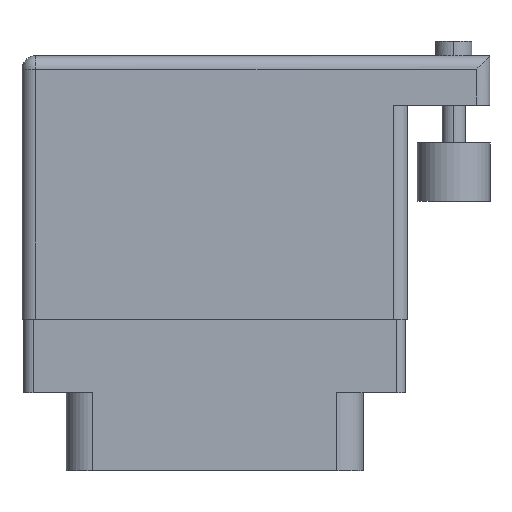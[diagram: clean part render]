
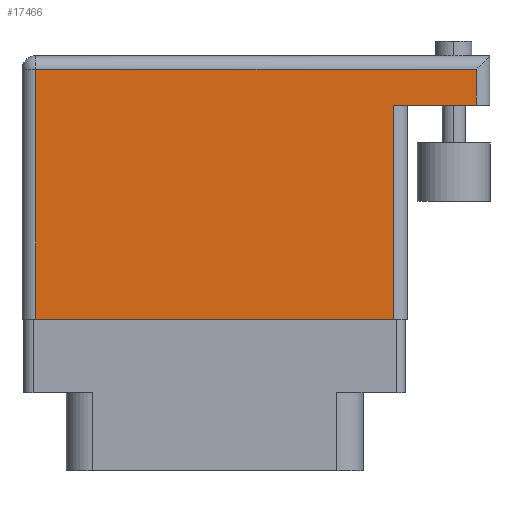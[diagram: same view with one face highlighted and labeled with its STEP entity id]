
A CAD part, front view. The second image highlights one B-rep face of the part: STEP entity #17466.
In plain terms, the highlighted face is planar.
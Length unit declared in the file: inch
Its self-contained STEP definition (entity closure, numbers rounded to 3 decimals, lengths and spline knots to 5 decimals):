
#4 = ORIENTED_EDGE ( 'NONE', *, *, #3222, .T. ) ;
#119 = DIRECTION ( 'NONE',  ( -1., 0., 0. ) ) ;
#309 = LINE ( 'NONE', #24208, #13355 ) ;
#433 = LINE ( 'NONE', #7741, #1077 ) ;
#990 = CARTESIAN_POINT ( 'NONE',  ( 1.562, 0.859, 0. ) ) ;
#1077 = VECTOR ( 'NONE', #3907, 39.37008 ) ;
#1354 = CARTESIAN_POINT ( 'NONE',  ( 1.609, 0.736, 0. ) ) ;
#1380 = CARTESIAN_POINT ( 'NONE',  ( 0., 0., 0. ) ) ;
#1875 = VECTOR ( 'NONE', #16314, 39.37008 ) ;
#2774 = DIRECTION ( 'NONE',  ( 0., 0., -1. ) ) ;
#3222 = EDGE_CURVE ( 'NONE', #6433, #5989, #10558, .T. ) ;
#3278 = ORIENTED_EDGE ( 'NONE', *, *, #6228, .T. ) ;
#3907 = DIRECTION ( 'NONE',  ( 0., -1., 0. ) ) ;
#4564 = PLANE ( 'NONE',  #9302 ) ;
#5813 = VECTOR ( 'NONE', #10812, 39.37008 ) ;
#5989 = VERTEX_POINT ( 'NONE', #990 ) ;
#6154 = EDGE_CURVE ( 'NONE', #6433, #10417, #8744, .T. ) ;
#6228 = EDGE_CURVE ( 'NONE', #17178, #23365, #433, .T. ) ;
#6433 = VERTEX_POINT ( 'NONE', #22819 ) ;
#7741 = CARTESIAN_POINT ( 'NONE',  ( 0.047, 0., 0. ) ) ;
#8744 = LINE ( 'NONE', #1354, #16030 ) ;
#8870 = ORIENTED_EDGE ( 'NONE', *, *, #23609, .T. ) ;
#9105 = EDGE_CURVE ( 'NONE', #5989, #17178, #309, .T. ) ;
#9302 = AXIS2_PLACEMENT_3D ( 'NONE', #12828, #2774, #24795 ) ;
#9848 = CARTESIAN_POINT ( 'NONE',  ( 1.278, 0., 0. ) ) ;
#10344 = CARTESIAN_POINT ( 'NONE',  ( 1.278, 0.736, 0. ) ) ;
#10417 = VERTEX_POINT ( 'NONE', #17077 ) ;
#10509 = ORIENTED_EDGE ( 'NONE', *, *, #9105, .T. ) ;
#10558 = LINE ( 'NONE', #16950, #5813 ) ;
#10812 = DIRECTION ( 'NONE',  ( 0., 1., 0. ) ) ;
#11589 = EDGE_LOOP ( 'NONE', ( #18604, #8870, #24326, #4, #10509, #3278 ) ) ;
#12704 = LINE ( 'NONE', #10344, #1875 ) ;
#12828 = CARTESIAN_POINT ( 'NONE',  ( 0., 0.906, 0. ) ) ;
#13355 = VECTOR ( 'NONE', #119, 39.37008 ) ;
#13416 = CARTESIAN_POINT ( 'NONE',  ( 0.047, 0., 0. ) ) ;
#15413 = DIRECTION ( 'NONE',  ( 1., 0., 0. ) ) ;
#16030 = VECTOR ( 'NONE', #19733, 39.37008 ) ;
#16314 = DIRECTION ( 'NONE',  ( 0., 1., 0. ) ) ;
#16950 = CARTESIAN_POINT ( 'NONE',  ( 1.562, 0.906, 0. ) ) ;
#17077 = CARTESIAN_POINT ( 'NONE',  ( 1.278, 0.736, 0. ) ) ;
#17178 = VERTEX_POINT ( 'NONE', #19935 ) ;
#17466 = ADVANCED_FACE ( 'NONE', ( #19651 ), #4564, .F. ) ;
#18604 = ORIENTED_EDGE ( 'NONE', *, *, #18943, .T. ) ;
#18943 = EDGE_CURVE ( 'NONE', #23365, #19583, #23318, .T. ) ;
#19583 = VERTEX_POINT ( 'NONE', #9848 ) ;
#19651 = FACE_OUTER_BOUND ( 'NONE', #11589, .T. ) ;
#19733 = DIRECTION ( 'NONE',  ( -1., 0., 0. ) ) ;
#19935 = CARTESIAN_POINT ( 'NONE',  ( 0.047, 0.859, 0. ) ) ;
#22819 = CARTESIAN_POINT ( 'NONE',  ( 1.562, 0.736, 0. ) ) ;
#23318 = LINE ( 'NONE', #1380, #23922 ) ;
#23365 = VERTEX_POINT ( 'NONE', #13416 ) ;
#23609 = EDGE_CURVE ( 'NONE', #19583, #10417, #12704, .T. ) ;
#23922 = VECTOR ( 'NONE', #15413, 39.37008 ) ;
#24208 = CARTESIAN_POINT ( 'NONE',  ( 0., 0.859, 0. ) ) ;
#24326 = ORIENTED_EDGE ( 'NONE', *, *, #6154, .F. ) ;
#24795 = DIRECTION ( 'NONE',  ( -1., 0., 0. ) ) ;
